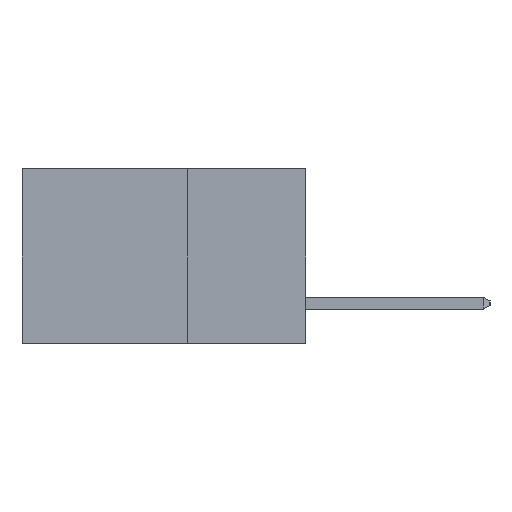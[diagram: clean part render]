
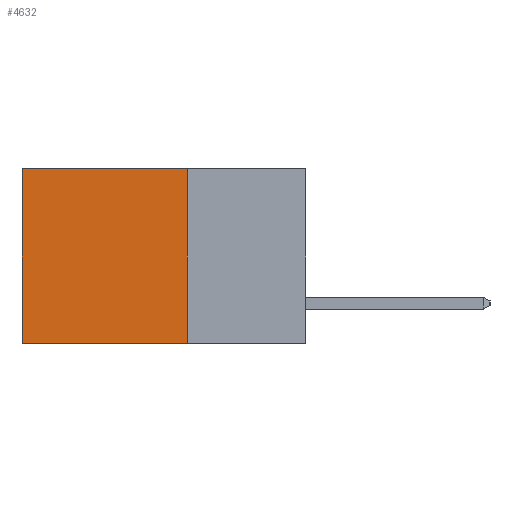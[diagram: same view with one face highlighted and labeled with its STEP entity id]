
A CAD part, left-side view. The second image highlights one B-rep face of the part: STEP entity #4632.
In plain terms, the highlighted planar face has unit normal (-1, 0, 0).
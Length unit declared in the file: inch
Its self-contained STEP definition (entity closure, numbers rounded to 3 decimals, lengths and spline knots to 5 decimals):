
#597 = DIRECTION ( 'NONE',  ( 0., 0., -1. ) ) ;
#931 = DIRECTION ( 'NONE',  ( 0., 0., -1. ) ) ;
#1800 = DIRECTION ( 'NONE',  ( 0., 1., 0. ) ) ;
#1870 = ORIENTED_EDGE ( 'NONE', *, *, #4967, .T. ) ;
#2424 = VECTOR ( 'NONE', #1800, 39.37008 ) ;
#2638 = VERTEX_POINT ( 'NONE', #7472 ) ;
#2788 = CARTESIAN_POINT ( 'NONE',  ( 0.2615, 0.25, -0.37 ) ) ;
#3269 = EDGE_CURVE ( 'NONE', #2638, #12405, #11856, .T. ) ;
#3950 = EDGE_CURVE ( 'NONE', #11321, #7329, #12169, .T. ) ;
#4309 = VECTOR ( 'NONE', #597, 39.37008 ) ;
#4632 = ADVANCED_FACE ( 'NONE', ( #11948 ), #10541, .F. ) ;
#4685 = CARTESIAN_POINT ( 'NONE',  ( 0.2615, 0.6, 0. ) ) ;
#4967 = EDGE_CURVE ( 'NONE', #2638, #11321, #16643, .T. ) ;
#6198 = EDGE_CURVE ( 'NONE', #12405, #7329, #13498, .T. ) ;
#7240 = CARTESIAN_POINT ( 'NONE',  ( 0.2615, 0.25, -0.37 ) ) ;
#7329 = VERTEX_POINT ( 'NONE', #12257 ) ;
#7472 = CARTESIAN_POINT ( 'NONE',  ( 0.2615, 0.25, 0. ) ) ;
#7820 = CARTESIAN_POINT ( 'NONE',  ( 0.2615, 0.25, -0.37 ) ) ;
#8478 = ORIENTED_EDGE ( 'NONE', *, *, #3950, .T. ) ;
#9679 = VECTOR ( 'NONE', #13862, 39.37008 ) ;
#10541 = PLANE ( 'NONE',  #14527 ) ;
#11308 = CARTESIAN_POINT ( 'NONE',  ( 0.2615, 0.25, -0.37 ) ) ;
#11321 = VERTEX_POINT ( 'NONE', #4685 ) ;
#11494 = ORIENTED_EDGE ( 'NONE', *, *, #6198, .F. ) ;
#11856 = LINE ( 'NONE', #11308, #4309 ) ;
#11948 = FACE_OUTER_BOUND ( 'NONE', #14721, .T. ) ;
#12169 = LINE ( 'NONE', #16882, #15259 ) ;
#12257 = CARTESIAN_POINT ( 'NONE',  ( 0.2615, 0.6, -0.37 ) ) ;
#12405 = VERTEX_POINT ( 'NONE', #2788 ) ;
#12567 = CARTESIAN_POINT ( 'NONE',  ( 0.2615, 0.25, 0. ) ) ;
#13140 = DIRECTION ( 'NONE',  ( 0., 0., -1. ) ) ;
#13498 = LINE ( 'NONE', #7240, #2424 ) ;
#13862 = DIRECTION ( 'NONE',  ( 0., 1., 0. ) ) ;
#13974 = ORIENTED_EDGE ( 'NONE', *, *, #3269, .F. ) ;
#14527 = AXIS2_PLACEMENT_3D ( 'NONE', #7820, #15735, #13140 ) ;
#14721 = EDGE_LOOP ( 'NONE', ( #8478, #11494, #13974, #1870 ) ) ;
#15259 = VECTOR ( 'NONE', #931, 39.37008 ) ;
#15735 = DIRECTION ( 'NONE',  ( 1., 0., 0. ) ) ;
#16643 = LINE ( 'NONE', #12567, #9679 ) ;
#16882 = CARTESIAN_POINT ( 'NONE',  ( 0.2615, 0.6, -0.37 ) ) ;
